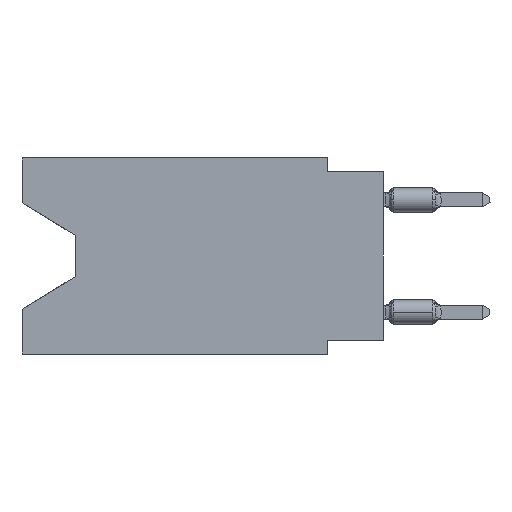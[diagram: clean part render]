
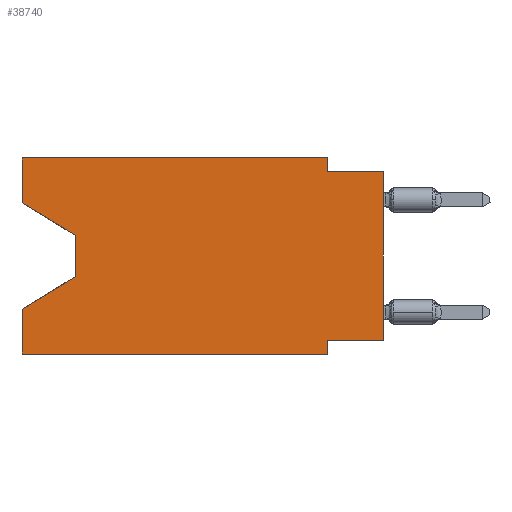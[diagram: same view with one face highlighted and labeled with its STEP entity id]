
A CAD part, left-side view. The second image highlights one B-rep face of the part: STEP entity #38740.
In plain terms, the highlighted planar face has unit normal (-1, 0, 0).
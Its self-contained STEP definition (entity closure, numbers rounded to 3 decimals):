
#442 = CARTESIAN_POINT ( 'NONE',  ( 0., 0., -0.635 ) ) ;
#1033 = DIRECTION ( 'NONE',  ( 1., 0., 0. ) ) ;
#1301 = PLANE ( 'NONE',  #7616 ) ;
#1876 = CARTESIAN_POINT ( 'NONE',  ( 0., 0., 0. ) ) ;
#2548 = DIRECTION ( 'NONE',  ( 0., 0., 1. ) ) ;
#3345 = CARTESIAN_POINT ( 'NONE',  ( 0., 16.383, 0. ) ) ;
#3407 = CARTESIAN_POINT ( 'NONE',  ( 0., 16.383, 0. ) ) ;
#3490 = ORIENTED_EDGE ( 'NONE', *, *, #29029, .F. ) ;
#4702 = VERTEX_POINT ( 'NONE', #31461 ) ;
#5039 = EDGE_CURVE ( 'NONE', #8832, #43418, #30867, .T. ) ;
#5511 = ORIENTED_EDGE ( 'NONE', *, *, #39527, .F. ) ;
#6276 = EDGE_CURVE ( 'NONE', #47081, #7328, #37703, .T. ) ;
#6472 = VECTOR ( 'NONE', #18192, 1000. ) ;
#7210 = LINE ( 'NONE', #23694, #23202 ) ;
#7328 = VERTEX_POINT ( 'NONE', #34798 ) ;
#7553 = ORIENTED_EDGE ( 'NONE', *, *, #8948, .F. ) ;
#7616 = AXIS2_PLACEMENT_3D ( 'NONE', #45646, #1033, #42124 ) ;
#8832 = VERTEX_POINT ( 'NONE', #14989 ) ;
#8948 = EDGE_CURVE ( 'NONE', #47410, #30723, #24408, .T. ) ;
#9060 = CARTESIAN_POINT ( 'NONE',  ( 0., 0., -8.255 ) ) ;
#9239 = VECTOR ( 'NONE', #2548, 1000. ) ;
#9300 = ORIENTED_EDGE ( 'NONE', *, *, #37865, .F. ) ;
#10014 = DIRECTION ( 'NONE',  ( 0., 1., 0. ) ) ;
#10564 = VECTOR ( 'NONE', #38103, 1000. ) ;
#11799 = DIRECTION ( 'NONE',  ( 0., -1., 0. ) ) ;
#14315 = ORIENTED_EDGE ( 'NONE', *, *, #6276, .T. ) ;
#14824 = ORIENTED_EDGE ( 'NONE', *, *, #32206, .F. ) ;
#14989 = CARTESIAN_POINT ( 'NONE',  ( 0., 2.54, -8.255 ) ) ;
#15089 = EDGE_CURVE ( 'NONE', #52305, #31076, #19965, .T. ) ;
#15486 = CARTESIAN_POINT ( 'NONE',  ( 0., 2.54, -8.89 ) ) ;
#15815 = EDGE_LOOP ( 'NONE', ( #14315, #44729, #50127, #14824, #51016, #20198, #3490, #47143, #5511, #7553, #30997, #9300 ) ) ;
#16117 = LINE ( 'NONE', #3407, #20991 ) ;
#17617 = EDGE_CURVE ( 'NONE', #19266, #4702, #18113, .T. ) ;
#18113 = LINE ( 'NONE', #1876, #10564 ) ;
#18192 = DIRECTION ( 'NONE',  ( 0., 0., -1. ) ) ;
#19206 = EDGE_CURVE ( 'NONE', #21992, #47410, #16117, .T. ) ;
#19266 = VERTEX_POINT ( 'NONE', #9060 ) ;
#19641 = DIRECTION ( 'NONE',  ( 0., 0., -1. ) ) ;
#19965 = LINE ( 'NONE', #20484, #46586 ) ;
#20198 = ORIENTED_EDGE ( 'NONE', *, *, #5039, .F. ) ;
#20484 = CARTESIAN_POINT ( 'NONE',  ( 0., 13.97, -5.385 ) ) ;
#20991 = VECTOR ( 'NONE', #11799, 1000. ) ;
#21465 = VECTOR ( 'NONE', #33143, 1000. ) ;
#21520 = LINE ( 'NONE', #442, #21465 ) ;
#21992 = VERTEX_POINT ( 'NONE', #28227 ) ;
#22019 = VECTOR ( 'NONE', #10014, 1000. ) ;
#23202 = VECTOR ( 'NONE', #40176, 1000. ) ;
#23694 = CARTESIAN_POINT ( 'NONE',  ( 0., 16.383, 0. ) ) ;
#24408 = LINE ( 'NONE', #36576, #50812 ) ;
#26689 = EDGE_CURVE ( 'NONE', #32163, #43418, #28938, .T. ) ;
#28227 = CARTESIAN_POINT ( 'NONE',  ( 0., 16.383, 0. ) ) ;
#28471 = LINE ( 'NONE', #3345, #9239 ) ;
#28938 = LINE ( 'NONE', #37057, #46447 ) ;
#28993 = DIRECTION ( 'NONE',  ( 0., 0., -1. ) ) ;
#29029 = EDGE_CURVE ( 'NONE', #19266, #8832, #51111, .T. ) ;
#29687 = EDGE_CURVE ( 'NONE', #7328, #52305, #32328, .T. ) ;
#30723 = VERTEX_POINT ( 'NONE', #42463 ) ;
#30867 = LINE ( 'NONE', #42781, #6472 ) ;
#30997 = ORIENTED_EDGE ( 'NONE', *, *, #19206, .F. ) ;
#31076 = VERTEX_POINT ( 'NONE', #42861 ) ;
#31461 = CARTESIAN_POINT ( 'NONE',  ( 0., 0., -0.635 ) ) ;
#32163 = VERTEX_POINT ( 'NONE', #42583 ) ;
#32206 = EDGE_CURVE ( 'NONE', #32163, #31076, #28471, .T. ) ;
#32328 = LINE ( 'NONE', #48841, #35898 ) ;
#32463 = VECTOR ( 'NONE', #45828, 1000. ) ;
#33143 = DIRECTION ( 'NONE',  ( 0., -1., 0. ) ) ;
#34798 = CARTESIAN_POINT ( 'NONE',  ( 0., 13.97, -3.505 ) ) ;
#35898 = VECTOR ( 'NONE', #19641, 1000. ) ;
#36576 = CARTESIAN_POINT ( 'NONE',  ( 0., 2.54, 0. ) ) ;
#36706 = DIRECTION ( 'NONE',  ( 0., 0.855, -0.519 ) ) ;
#37057 = CARTESIAN_POINT ( 'NONE',  ( 0., 16.383, -8.89 ) ) ;
#37703 = LINE ( 'NONE', #49626, #32463 ) ;
#37865 = EDGE_CURVE ( 'NONE', #47081, #21992, #7210, .T. ) ;
#38103 = DIRECTION ( 'NONE',  ( 0., 0., 1. ) ) ;
#38740 = ADVANCED_FACE ( 'NONE', ( #45912 ), #1301, .F. ) ;
#39527 = EDGE_CURVE ( 'NONE', #30723, #4702, #21520, .T. ) ;
#40176 = DIRECTION ( 'NONE',  ( 0., 0., 1. ) ) ;
#41386 = DIRECTION ( 'NONE',  ( 0., -1., 0. ) ) ;
#41448 = CARTESIAN_POINT ( 'NONE',  ( 0., 13.97, -5.385 ) ) ;
#42124 = DIRECTION ( 'NONE',  ( 0., 0., -1. ) ) ;
#42463 = CARTESIAN_POINT ( 'NONE',  ( 0., 2.54, -0.635 ) ) ;
#42583 = CARTESIAN_POINT ( 'NONE',  ( 0., 16.383, -8.89 ) ) ;
#42781 = CARTESIAN_POINT ( 'NONE',  ( 0., 2.54, -8.89 ) ) ;
#42861 = CARTESIAN_POINT ( 'NONE',  ( 0., 16.383, -6.852 ) ) ;
#43418 = VERTEX_POINT ( 'NONE', #15486 ) ;
#44729 = ORIENTED_EDGE ( 'NONE', *, *, #29687, .T. ) ;
#45646 = CARTESIAN_POINT ( 'NONE',  ( 0., 16.383, 0. ) ) ;
#45828 = DIRECTION ( 'NONE',  ( 0., -0.855, -0.519 ) ) ;
#45912 = FACE_OUTER_BOUND ( 'NONE', #15815, .T. ) ;
#46194 = CARTESIAN_POINT ( 'NONE',  ( 0., 2.54, 0. ) ) ;
#46447 = VECTOR ( 'NONE', #41386, 1000. ) ;
#46586 = VECTOR ( 'NONE', #36706, 1000. ) ;
#47081 = VERTEX_POINT ( 'NONE', #50560 ) ;
#47143 = ORIENTED_EDGE ( 'NONE', *, *, #17617, .T. ) ;
#47301 = CARTESIAN_POINT ( 'NONE',  ( 0., 0., -8.255 ) ) ;
#47410 = VERTEX_POINT ( 'NONE', #46194 ) ;
#48841 = CARTESIAN_POINT ( 'NONE',  ( 0., 13.97, -3.505 ) ) ;
#49626 = CARTESIAN_POINT ( 'NONE',  ( 0., 16.383, -2.038 ) ) ;
#50127 = ORIENTED_EDGE ( 'NONE', *, *, #15089, .T. ) ;
#50560 = CARTESIAN_POINT ( 'NONE',  ( 0., 16.383, -2.038 ) ) ;
#50812 = VECTOR ( 'NONE', #28993, 1000. ) ;
#51016 = ORIENTED_EDGE ( 'NONE', *, *, #26689, .T. ) ;
#51111 = LINE ( 'NONE', #47301, #22019 ) ;
#52305 = VERTEX_POINT ( 'NONE', #41448 ) ;
